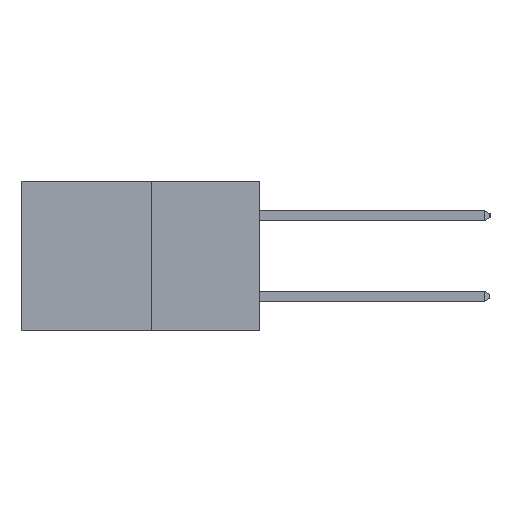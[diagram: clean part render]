
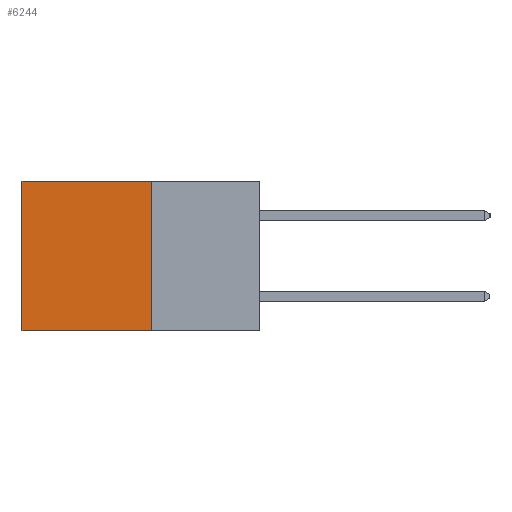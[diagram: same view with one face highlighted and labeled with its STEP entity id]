
A CAD part, left-side view. The second image highlights one B-rep face of the part: STEP entity #6244.
In plain terms, the highlighted planar face has unit normal (-1, 0, 0).
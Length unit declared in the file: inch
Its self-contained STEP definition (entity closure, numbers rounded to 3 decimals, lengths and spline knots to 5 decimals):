
#499 = LINE ( 'NONE', #12347, #13448 ) ;
#566 = CARTESIAN_POINT ( 'NONE',  ( 0.277, 0.59, -0.37 ) ) ;
#1338 = CARTESIAN_POINT ( 'NONE',  ( 0.277, 0.27, 0. ) ) ;
#1408 = CARTESIAN_POINT ( 'NONE',  ( 0.277, 0.59, 0. ) ) ;
#1840 = DIRECTION ( 'NONE',  ( 0., 0., -1. ) ) ;
#2033 = CARTESIAN_POINT ( 'NONE',  ( 0.277, 0.27, -0.37 ) ) ;
#2518 = VERTEX_POINT ( 'NONE', #14316 ) ;
#4092 = EDGE_CURVE ( 'NONE', #2518, #5748, #6874, .T. ) ;
#4608 = ORIENTED_EDGE ( 'NONE', *, *, #8564, .T. ) ;
#4740 = ORIENTED_EDGE ( 'NONE', *, *, #9157, .F. ) ;
#4821 = VECTOR ( 'NONE', #12190, 39.37008 ) ;
#5052 = ORIENTED_EDGE ( 'NONE', *, *, #4092, .F. ) ;
#5066 = ORIENTED_EDGE ( 'NONE', *, *, #10659, .T. ) ;
#5748 = VERTEX_POINT ( 'NONE', #10555 ) ;
#6244 = ADVANCED_FACE ( 'NONE', ( #9854 ), #6792, .F. ) ;
#6603 = CARTESIAN_POINT ( 'NONE',  ( 0.277, 0.59, -0.37 ) ) ;
#6722 = DIRECTION ( 'NONE',  ( 0., 0., -1. ) ) ;
#6744 = DIRECTION ( 'NONE',  ( 1., 0., 0. ) ) ;
#6791 = CARTESIAN_POINT ( 'NONE',  ( 0.277, 0.27, -0.37 ) ) ;
#6792 = PLANE ( 'NONE',  #10164 ) ;
#6874 = LINE ( 'NONE', #2033, #12633 ) ;
#7389 = LINE ( 'NONE', #1338, #9842 ) ;
#7608 = VERTEX_POINT ( 'NONE', #6603 ) ;
#8382 = DIRECTION ( 'NONE',  ( 0., 1., 0. ) ) ;
#8564 = EDGE_CURVE ( 'NONE', #10595, #7608, #11490, .T. ) ;
#9038 = DIRECTION ( 'NONE',  ( 0., 1., 0. ) ) ;
#9157 = EDGE_CURVE ( 'NONE', #5748, #7608, #499, .T. ) ;
#9842 = VECTOR ( 'NONE', #8382, 39.37008 ) ;
#9854 = FACE_OUTER_BOUND ( 'NONE', #14603, .T. ) ;
#10164 = AXIS2_PLACEMENT_3D ( 'NONE', #6791, #6744, #6722 ) ;
#10555 = CARTESIAN_POINT ( 'NONE',  ( 0.277, 0.27, -0.37 ) ) ;
#10595 = VERTEX_POINT ( 'NONE', #1408 ) ;
#10659 = EDGE_CURVE ( 'NONE', #2518, #10595, #7389, .T. ) ;
#11490 = LINE ( 'NONE', #566, #4821 ) ;
#12190 = DIRECTION ( 'NONE',  ( 0., 0., -1. ) ) ;
#12347 = CARTESIAN_POINT ( 'NONE',  ( 0.277, 0.27, -0.37 ) ) ;
#12633 = VECTOR ( 'NONE', #1840, 39.37008 ) ;
#13448 = VECTOR ( 'NONE', #9038, 39.37008 ) ;
#14316 = CARTESIAN_POINT ( 'NONE',  ( 0.277, 0.27, 0. ) ) ;
#14603 = EDGE_LOOP ( 'NONE', ( #4608, #4740, #5052, #5066 ) ) ;
